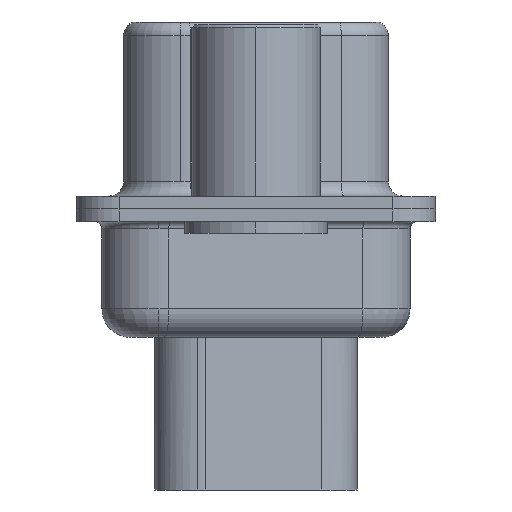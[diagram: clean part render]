
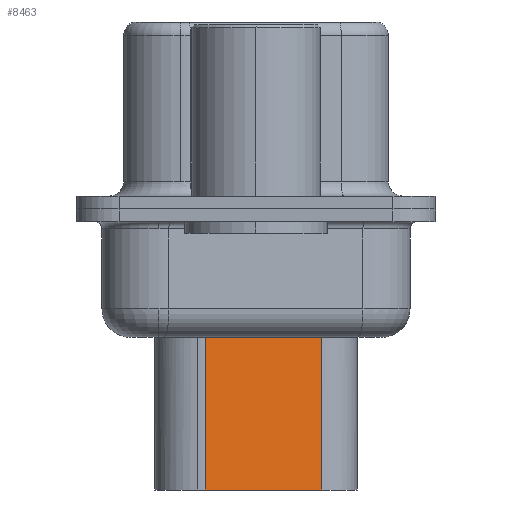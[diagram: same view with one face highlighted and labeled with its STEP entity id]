
A CAD part, left-side view. The second image highlights one B-rep face of the part: STEP entity #8463.
In plain terms, the highlighted planar face has unit normal (-0.985, -0.174, 0).
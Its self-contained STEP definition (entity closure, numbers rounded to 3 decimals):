
#192 = CARTESIAN_POINT ( 'NONE',  ( 5.238, -2.3, -9.85 ) ) ;
#851 = CARTESIAN_POINT ( 'NONE',  ( 5.238, -2.3, -3.1 ) ) ;
#959 = EDGE_CURVE ( 'NONE', #2643, #12676, #11972, .T. ) ;
#1836 = EDGE_LOOP ( 'NONE', ( #2587, #12937, #11274, #13442 ) ) ;
#2186 = DIRECTION ( 'NONE',  ( -0.985, -0.174, 0. ) ) ;
#2318 = CARTESIAN_POINT ( 'NONE',  ( 4.519, 1.78, -3.1 ) ) ;
#2587 = ORIENTED_EDGE ( 'NONE', *, *, #959, .F. ) ;
#2608 = VECTOR ( 'NONE', #8880, 1000. ) ;
#2643 = VERTEX_POINT ( 'NONE', #11295 ) ;
#3026 = VECTOR ( 'NONE', #8494, 1000. ) ;
#4120 = AXIS2_PLACEMENT_3D ( 'NONE', #9750, #2186, #14176 ) ;
#4351 = PLANE ( 'NONE',  #4120 ) ;
#5444 = FACE_OUTER_BOUND ( 'NONE', #1836, .T. ) ;
#5826 = LINE ( 'NONE', #10282, #2608 ) ;
#6522 = LINE ( 'NONE', #2318, #13041 ) ;
#6765 = CARTESIAN_POINT ( 'NONE',  ( 4.519, 1.78, -9.85 ) ) ;
#7321 = VERTEX_POINT ( 'NONE', #6765 ) ;
#8463 = ADVANCED_FACE ( 'NONE', ( #5444 ), #4351, .T. ) ;
#8494 = DIRECTION ( 'NONE',  ( 0., 0., -1. ) ) ;
#8769 = CARTESIAN_POINT ( 'NONE',  ( 4.519, 1.78, -3.975 ) ) ;
#8880 = DIRECTION ( 'NONE',  ( -0.174, 0.985, 0. ) ) ;
#9750 = CARTESIAN_POINT ( 'NONE',  ( 4.519, 1.78, -3.1 ) ) ;
#10185 = VECTOR ( 'NONE', #10501, 1000. ) ;
#10199 = EDGE_CURVE ( 'NONE', #12490, #7321, #6522, .T. ) ;
#10282 = CARTESIAN_POINT ( 'NONE',  ( 4.348, 2.749, -3.975 ) ) ;
#10501 = DIRECTION ( 'NONE',  ( -0.174, 0.985, 0. ) ) ;
#10710 = LINE ( 'NONE', #13915, #10185 ) ;
#11260 = EDGE_CURVE ( 'NONE', #2643, #12490, #5826, .T. ) ;
#11274 = ORIENTED_EDGE ( 'NONE', *, *, #10199, .T. ) ;
#11295 = CARTESIAN_POINT ( 'NONE',  ( 5.238, -2.3, -3.975 ) ) ;
#11972 = LINE ( 'NONE', #851, #3026 ) ;
#12134 = DIRECTION ( 'NONE',  ( 0., 0., -1. ) ) ;
#12490 = VERTEX_POINT ( 'NONE', #8769 ) ;
#12676 = VERTEX_POINT ( 'NONE', #192 ) ;
#12937 = ORIENTED_EDGE ( 'NONE', *, *, #11260, .T. ) ;
#13041 = VECTOR ( 'NONE', #12134, 1000. ) ;
#13442 = ORIENTED_EDGE ( 'NONE', *, *, #13588, .F. ) ;
#13588 = EDGE_CURVE ( 'NONE', #12676, #7321, #10710, .T. ) ;
#13915 = CARTESIAN_POINT ( 'NONE',  ( 4.519, 1.78, -9.85 ) ) ;
#14176 = DIRECTION ( 'NONE',  ( 0.174, -0.985, 0. ) ) ;
